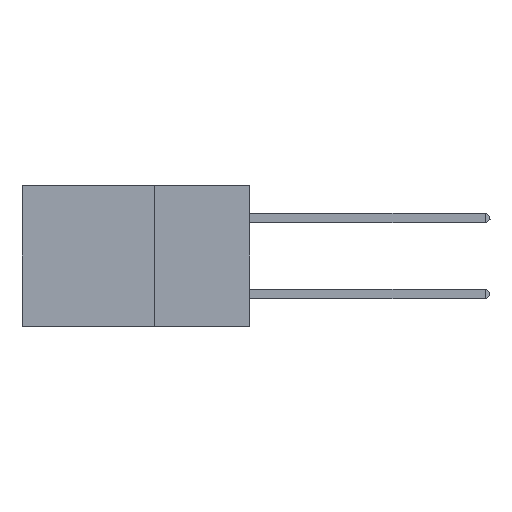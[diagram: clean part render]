
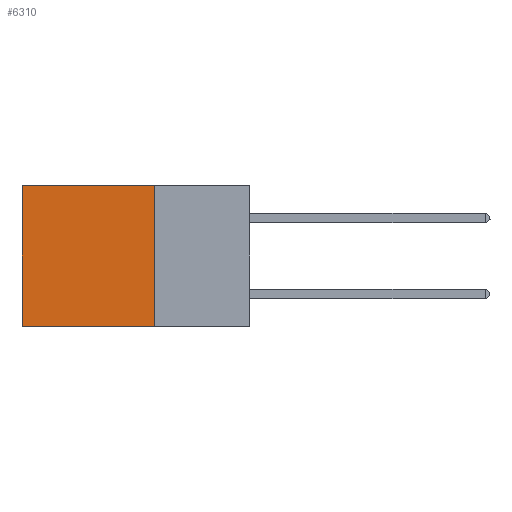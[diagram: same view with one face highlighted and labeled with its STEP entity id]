
A CAD part, left-side view. The second image highlights one B-rep face of the part: STEP entity #6310.
In plain terms, the highlighted planar face has unit normal (-1, 0, 0).
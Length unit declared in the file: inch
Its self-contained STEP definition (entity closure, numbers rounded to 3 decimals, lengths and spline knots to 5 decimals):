
#692 = AXIS2_PLACEMENT_3D ( 'NONE', #19796, #22665, #13739 ) ;
#876 = VERTEX_POINT ( 'NONE', #14736 ) ;
#1194 = CARTESIAN_POINT ( 'NONE',  ( 0.2875, 0.25, 0. ) ) ;
#1481 = ORIENTED_EDGE ( 'NONE', *, *, #7704, .F. ) ;
#1630 = CARTESIAN_POINT ( 'NONE',  ( 0.2875, 0.25, -0.37 ) ) ;
#5101 = VECTOR ( 'NONE', #26170, 39.37008 ) ;
#6310 = ADVANCED_FACE ( 'NONE', ( #8536 ), #30198, .F. ) ;
#7067 = VERTEX_POINT ( 'NONE', #10800 ) ;
#7704 = EDGE_CURVE ( 'NONE', #9772, #876, #8142, .T. ) ;
#8132 = ORIENTED_EDGE ( 'NONE', *, *, #14038, .T. ) ;
#8142 = LINE ( 'NONE', #18889, #18023 ) ;
#8536 = FACE_OUTER_BOUND ( 'NONE', #31483, .T. ) ;
#9512 = LINE ( 'NONE', #23477, #5101 ) ;
#9772 = VERTEX_POINT ( 'NONE', #1630 ) ;
#10800 = CARTESIAN_POINT ( 'NONE',  ( 0.2875, 0.6, 0. ) ) ;
#13739 = DIRECTION ( 'NONE',  ( 0., 0., -1. ) ) ;
#13953 = VERTEX_POINT ( 'NONE', #28820 ) ;
#14038 = EDGE_CURVE ( 'NONE', #13953, #7067, #16089, .T. ) ;
#14736 = CARTESIAN_POINT ( 'NONE',  ( 0.2875, 0.6, -0.37 ) ) ;
#15855 = DIRECTION ( 'NONE',  ( 0., 1., 0. ) ) ;
#16089 = LINE ( 'NONE', #19317, #18492 ) ;
#18023 = VECTOR ( 'NONE', #15855, 39.37008 ) ;
#18492 = VECTOR ( 'NONE', #27187, 39.37008 ) ;
#18889 = CARTESIAN_POINT ( 'NONE',  ( 0.2875, 0.25, -0.37 ) ) ;
#19317 = CARTESIAN_POINT ( 'NONE',  ( 0.2875, 0.25, 0. ) ) ;
#19796 = CARTESIAN_POINT ( 'NONE',  ( 0.2875, 0.25, 0. ) ) ;
#19997 = DIRECTION ( 'NONE',  ( 0., 0., -1. ) ) ;
#22665 = DIRECTION ( 'NONE',  ( 1., 0., 0. ) ) ;
#22689 = LINE ( 'NONE', #1194, #34439 ) ;
#23477 = CARTESIAN_POINT ( 'NONE',  ( 0.2875, 0.6, 0. ) ) ;
#25067 = ORIENTED_EDGE ( 'NONE', *, *, #35199, .F. ) ;
#26170 = DIRECTION ( 'NONE',  ( 0., 0., -1. ) ) ;
#27118 = EDGE_CURVE ( 'NONE', #7067, #876, #9512, .T. ) ;
#27187 = DIRECTION ( 'NONE',  ( 0., 1., 0. ) ) ;
#28820 = CARTESIAN_POINT ( 'NONE',  ( 0.2875, 0.25, 0. ) ) ;
#30198 = PLANE ( 'NONE',  #692 ) ;
#30660 = ORIENTED_EDGE ( 'NONE', *, *, #27118, .T. ) ;
#31483 = EDGE_LOOP ( 'NONE', ( #30660, #1481, #25067, #8132 ) ) ;
#34439 = VECTOR ( 'NONE', #19997, 39.37008 ) ;
#35199 = EDGE_CURVE ( 'NONE', #13953, #9772, #22689, .T. ) ;
